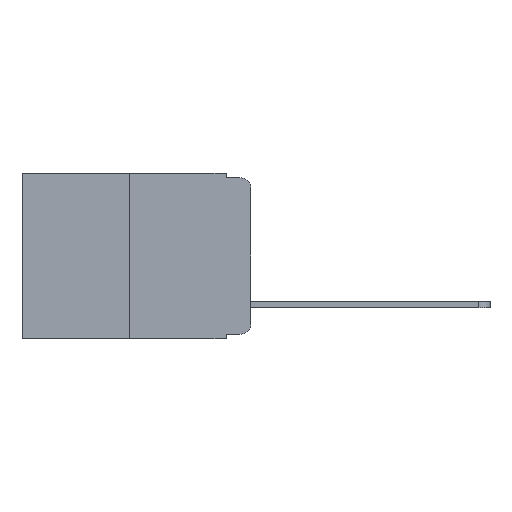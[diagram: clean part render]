
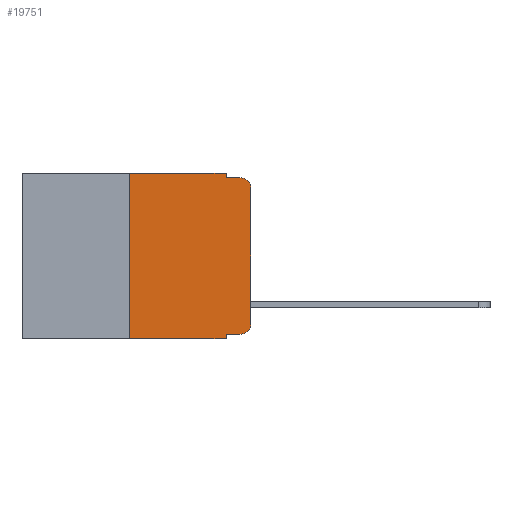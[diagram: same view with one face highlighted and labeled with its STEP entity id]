
A CAD part, left-side view. The second image highlights one B-rep face of the part: STEP entity #19751.
In plain terms, the highlighted planar face has unit normal (-1, 0, 0).
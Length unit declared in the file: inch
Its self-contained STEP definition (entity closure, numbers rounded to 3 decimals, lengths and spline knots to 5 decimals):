
#242 = VERTEX_POINT ( 'NONE', #9978 ) ;
#722 = VERTEX_POINT ( 'NONE', #24083 ) ;
#835 = ORIENTED_EDGE ( 'NONE', *, *, #14561, .T. ) ;
#924 = LINE ( 'NONE', #16000, #24143 ) ;
#993 = EDGE_CURVE ( 'NONE', #13061, #10889, #21559, .T. ) ;
#1311 = DIRECTION ( 'NONE',  ( 0., 0., -1. ) ) ;
#1560 = EDGE_CURVE ( 'NONE', #242, #7145, #12904, .T. ) ;
#1585 = DIRECTION ( 'NONE',  ( 0., -1., 0. ) ) ;
#1665 = CARTESIAN_POINT ( 'NONE',  ( 0., 0., 0. ) ) ;
#2647 = ORIENTED_EDGE ( 'NONE', *, *, #13883, .T. ) ;
#2659 = VECTOR ( 'NONE', #8273, 39.37008 ) ;
#2770 = ORIENTED_EDGE ( 'NONE', *, *, #1560, .F. ) ;
#2930 = FACE_OUTER_BOUND ( 'NONE', #3164, .T. ) ;
#3074 = EDGE_CURVE ( 'NONE', #13061, #22874, #924, .T. ) ;
#3164 = EDGE_LOOP ( 'NONE', ( #835, #17297, #23099, #2770, #20674, #16220, #15225, #19218, #6165, #2647 ) ) ;
#3395 = DIRECTION ( 'NONE',  ( 0., -1., 0. ) ) ;
#3477 = PLANE ( 'NONE',  #5435 ) ;
#4413 = DIRECTION ( 'NONE',  ( 0., -1., 0. ) ) ;
#4970 = EDGE_CURVE ( 'NONE', #7145, #21452, #8563, .T. ) ;
#5212 = CARTESIAN_POINT ( 'NONE',  ( 0., 0.02, -0.333 ) ) ;
#5399 = DIRECTION ( 'NONE',  ( 1., 0., 0. ) ) ;
#5435 = AXIS2_PLACEMENT_3D ( 'NONE', #16795, #5399, #22194 ) ;
#5867 = CARTESIAN_POINT ( 'NONE',  ( 0., 0.051, -0.333 ) ) ;
#5975 = CIRCLE ( 'NONE', #19645, 0.02 ) ;
#6133 = CARTESIAN_POINT ( 'NONE',  ( 0., 0.25, 0. ) ) ;
#6165 = ORIENTED_EDGE ( 'NONE', *, *, #993, .T. ) ;
#6703 = CARTESIAN_POINT ( 'NONE',  ( 0., 0.473, 0. ) ) ;
#6882 = CARTESIAN_POINT ( 'NONE',  ( 0., 0.02, -0.01 ) ) ;
#7145 = VERTEX_POINT ( 'NONE', #18393 ) ;
#7586 = VERTEX_POINT ( 'NONE', #24466 ) ;
#8273 = DIRECTION ( 'NONE',  ( 0., 0., 1. ) ) ;
#8543 = VERTEX_POINT ( 'NONE', #23325 ) ;
#8563 = LINE ( 'NONE', #13177, #16645 ) ;
#8721 = VECTOR ( 'NONE', #24636, 39.37008 ) ;
#8739 = DIRECTION ( 'NONE',  ( -1., 0., 0. ) ) ;
#9635 = VECTOR ( 'NONE', #11034, 39.37008 ) ;
#9800 = CARTESIAN_POINT ( 'NONE',  ( 0., 0.051, 0. ) ) ;
#9978 = CARTESIAN_POINT ( 'NONE',  ( 0., 0.051, 0. ) ) ;
#10610 = DIRECTION ( 'NONE',  ( -1., 0., 0. ) ) ;
#10889 = VERTEX_POINT ( 'NONE', #5212 ) ;
#11034 = DIRECTION ( 'NONE',  ( 0., 0., 1. ) ) ;
#11251 = EDGE_CURVE ( 'NONE', #8543, #22874, #17095, .T. ) ;
#11268 = LINE ( 'NONE', #6703, #21402 ) ;
#11986 = VECTOR ( 'NONE', #4413, 39.37008 ) ;
#12438 = DIRECTION ( 'NONE',  ( 0., 0., -1. ) ) ;
#12904 = LINE ( 'NONE', #9800, #8721 ) ;
#13061 = VERTEX_POINT ( 'NONE', #5867 ) ;
#13177 = CARTESIAN_POINT ( 'NONE',  ( 0., 0.051, -0.01 ) ) ;
#13883 = EDGE_CURVE ( 'NONE', #10889, #16813, #20128, .T. ) ;
#14561 = EDGE_CURVE ( 'NONE', #16813, #7586, #19769, .T. ) ;
#15225 = ORIENTED_EDGE ( 'NONE', *, *, #11251, .T. ) ;
#15979 = CARTESIAN_POINT ( 'NONE',  ( 0., 0., -0.313 ) ) ;
#16000 = CARTESIAN_POINT ( 'NONE',  ( 0., 0.051, 0. ) ) ;
#16008 = EDGE_CURVE ( 'NONE', #7586, #21452, #5975, .T. ) ;
#16077 = LINE ( 'NONE', #6133, #2659 ) ;
#16220 = ORIENTED_EDGE ( 'NONE', *, *, #23850, .F. ) ;
#16645 = VECTOR ( 'NONE', #3395, 39.37008 ) ;
#16795 = CARTESIAN_POINT ( 'NONE',  ( 0., 0.473, 0. ) ) ;
#16813 = VERTEX_POINT ( 'NONE', #15979 ) ;
#17095 = LINE ( 'NONE', #19171, #11986 ) ;
#17297 = ORIENTED_EDGE ( 'NONE', *, *, #16008, .T. ) ;
#17491 = CARTESIAN_POINT ( 'NONE',  ( 0., 0.051, -0.333 ) ) ;
#17622 = EDGE_CURVE ( 'NONE', #722, #242, #11268, .T. ) ;
#18393 = CARTESIAN_POINT ( 'NONE',  ( 0., 0.051, -0.01 ) ) ;
#19146 = AXIS2_PLACEMENT_3D ( 'NONE', #20187, #8739, #22082 ) ;
#19171 = CARTESIAN_POINT ( 'NONE',  ( 0., 0.473, -0.343 ) ) ;
#19218 = ORIENTED_EDGE ( 'NONE', *, *, #3074, .F. ) ;
#19491 = DIRECTION ( 'NONE',  ( 0., -1., 0. ) ) ;
#19645 = AXIS2_PLACEMENT_3D ( 'NONE', #20218, #10610, #12438 ) ;
#19751 = ADVANCED_FACE ( 'NONE', ( #2930 ), #3477, .F. ) ;
#19769 = LINE ( 'NONE', #1665, #9635 ) ;
#20128 = CIRCLE ( 'NONE', #19146, 0.02 ) ;
#20187 = CARTESIAN_POINT ( 'NONE',  ( 0., 0.02, -0.313 ) ) ;
#20218 = CARTESIAN_POINT ( 'NONE',  ( 0., 0.02, -0.03 ) ) ;
#20674 = ORIENTED_EDGE ( 'NONE', *, *, #17622, .F. ) ;
#20977 = VECTOR ( 'NONE', #19491, 39.37008 ) ;
#21402 = VECTOR ( 'NONE', #1585, 39.37008 ) ;
#21452 = VERTEX_POINT ( 'NONE', #6882 ) ;
#21559 = LINE ( 'NONE', #17491, #20977 ) ;
#22082 = DIRECTION ( 'NONE',  ( 0., 0., -1. ) ) ;
#22194 = DIRECTION ( 'NONE',  ( 0., 0., -1. ) ) ;
#22874 = VERTEX_POINT ( 'NONE', #24025 ) ;
#23099 = ORIENTED_EDGE ( 'NONE', *, *, #4970, .F. ) ;
#23325 = CARTESIAN_POINT ( 'NONE',  ( 0., 0.25, -0.343 ) ) ;
#23850 = EDGE_CURVE ( 'NONE', #8543, #722, #16077, .T. ) ;
#24025 = CARTESIAN_POINT ( 'NONE',  ( 0., 0.051, -0.343 ) ) ;
#24083 = CARTESIAN_POINT ( 'NONE',  ( 0., 0.25, 0. ) ) ;
#24143 = VECTOR ( 'NONE', #1311, 39.37008 ) ;
#24466 = CARTESIAN_POINT ( 'NONE',  ( 0., 0., -0.03 ) ) ;
#24636 = DIRECTION ( 'NONE',  ( 0., 0., -1. ) ) ;
